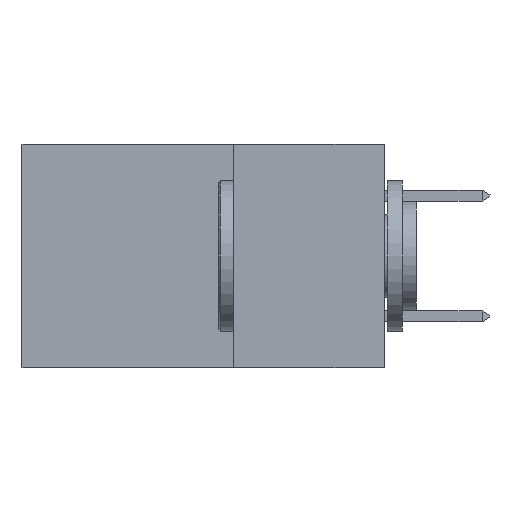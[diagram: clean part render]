
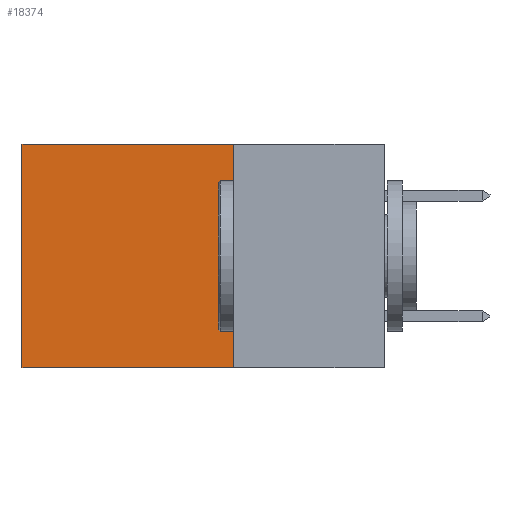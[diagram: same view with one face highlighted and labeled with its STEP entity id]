
A CAD part, left-side view. The second image highlights one B-rep face of the part: STEP entity #18374.
In plain terms, the highlighted planar face has unit normal (-1, 0, 0).
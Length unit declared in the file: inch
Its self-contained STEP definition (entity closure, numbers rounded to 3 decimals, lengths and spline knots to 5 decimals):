
#236 = CARTESIAN_POINT ( 'NONE',  ( 0.2875, 0.25, 0. ) ) ;
#1150 = FACE_OUTER_BOUND ( 'NONE', #17318, .T. ) ;
#1188 = CARTESIAN_POINT ( 'NONE',  ( 0.2875, 0.6, 0. ) ) ;
#2226 = DIRECTION ( 'NONE',  ( 0., 0., -1. ) ) ;
#2543 = CARTESIAN_POINT ( 'NONE',  ( 0.2875, 0.25, 0. ) ) ;
#2623 = ORIENTED_EDGE ( 'NONE', *, *, #9045, .T. ) ;
#2970 = ORIENTED_EDGE ( 'NONE', *, *, #12085, .F. ) ;
#3173 = DIRECTION ( 'NONE',  ( 0., 0., -1. ) ) ;
#3357 = VECTOR ( 'NONE', #22019, 39.37008 ) ;
#4573 = DIRECTION ( 'NONE',  ( 0., 0., -1. ) ) ;
#4670 = CARTESIAN_POINT ( 'NONE',  ( 0.2875, 0.6, 0. ) ) ;
#4910 = ORIENTED_EDGE ( 'NONE', *, *, #12353, .F. ) ;
#6466 = CARTESIAN_POINT ( 'NONE',  ( 0.2875, 0.25, 0. ) ) ;
#7835 = VERTEX_POINT ( 'NONE', #4670 ) ;
#7988 = VECTOR ( 'NONE', #16609, 39.37008 ) ;
#9045 = EDGE_CURVE ( 'NONE', #16665, #7835, #18951, .T. ) ;
#11619 = AXIS2_PLACEMENT_3D ( 'NONE', #2543, #16261, #4573 ) ;
#12085 = EDGE_CURVE ( 'NONE', #16665, #21637, #19847, .T. ) ;
#12353 = EDGE_CURVE ( 'NONE', #21637, #22340, #23463, .T. ) ;
#12354 = PLANE ( 'NONE',  #11619 ) ;
#14083 = VECTOR ( 'NONE', #2226, 39.37008 ) ;
#14667 = CARTESIAN_POINT ( 'NONE',  ( 0.2875, 0.25, -0.37 ) ) ;
#16261 = DIRECTION ( 'NONE',  ( 1., 0., 0. ) ) ;
#16400 = VECTOR ( 'NONE', #3173, 39.37008 ) ;
#16609 = DIRECTION ( 'NONE',  ( 0., 1., 0. ) ) ;
#16665 = VERTEX_POINT ( 'NONE', #17686 ) ;
#17001 = LINE ( 'NONE', #1188, #16400 ) ;
#17318 = EDGE_LOOP ( 'NONE', ( #18653, #4910, #2970, #2623 ) ) ;
#17686 = CARTESIAN_POINT ( 'NONE',  ( 0.2875, 0.25, 0. ) ) ;
#18374 = ADVANCED_FACE ( 'NONE', ( #1150 ), #12354, .F. ) ;
#18653 = ORIENTED_EDGE ( 'NONE', *, *, #19894, .T. ) ;
#18951 = LINE ( 'NONE', #6466, #3357 ) ;
#19847 = LINE ( 'NONE', #236, #14083 ) ;
#19894 = EDGE_CURVE ( 'NONE', #7835, #22340, #17001, .T. ) ;
#21637 = VERTEX_POINT ( 'NONE', #23415 ) ;
#22019 = DIRECTION ( 'NONE',  ( 0., 1., 0. ) ) ;
#22340 = VERTEX_POINT ( 'NONE', #23551 ) ;
#23415 = CARTESIAN_POINT ( 'NONE',  ( 0.2875, 0.25, -0.37 ) ) ;
#23463 = LINE ( 'NONE', #14667, #7988 ) ;
#23551 = CARTESIAN_POINT ( 'NONE',  ( 0.2875, 0.6, -0.37 ) ) ;
